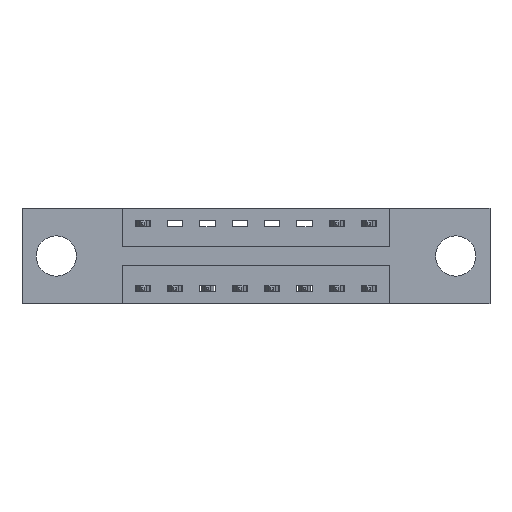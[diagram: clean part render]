
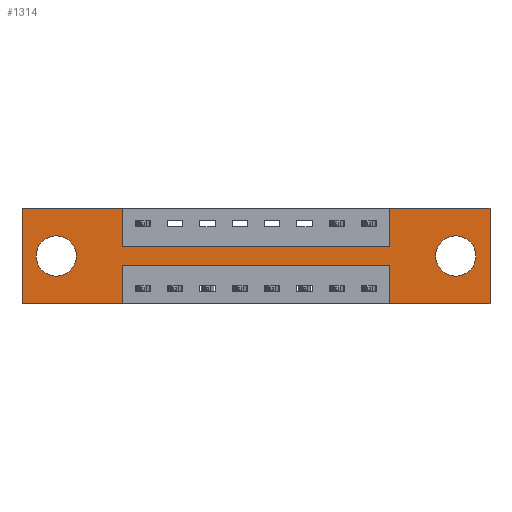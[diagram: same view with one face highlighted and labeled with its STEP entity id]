
A CAD part, front view. The second image highlights one B-rep face of the part: STEP entity #1314.
In plain terms, the highlighted planar face has unit normal (0, -1, 0).
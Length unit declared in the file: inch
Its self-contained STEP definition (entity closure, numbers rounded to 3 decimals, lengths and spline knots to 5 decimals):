
#1 = CARTESIAN_POINT ( 'NONE',  ( 1.4225, 0., 0. ) ) ;
#116 = CARTESIAN_POINT ( 'NONE',  ( 0., 0., 0. ) ) ;
#119 = EDGE_LOOP ( 'NONE', ( #2392, #2402 ) ) ;
#208 = VERTEX_POINT ( 'NONE', #7339 ) ;
#280 = CARTESIAN_POINT ( 'NONE',  ( 1.6775, 0., -0.185 ) ) ;
#337 = DIRECTION ( 'NONE',  ( 0., 1., 0. ) ) ;
#385 = EDGE_LOOP ( 'NONE', ( #2421, #2429, #2489, #2523, #2609, #2802, #2816, #2827, #2843, #3000, #3020, #3051 ) ) ;
#409 = CARTESIAN_POINT ( 'NONE',  ( 1.81, 0., -0.37 ) ) ;
#554 = LINE ( 'NONE', #9428, #5998 ) ;
#558 = DIRECTION ( 'NONE',  ( 0., 0., -1. ) ) ;
#704 = VECTOR ( 'NONE', #7779, 39.37008 ) ;
#785 = VECTOR ( 'NONE', #7935, 39.37008 ) ;
#791 = VERTEX_POINT ( 'NONE', #3571 ) ;
#1025 = CIRCLE ( 'NONE', #1212, 0.078 ) ;
#1055 = VECTOR ( 'NONE', #2573, 39.37008 ) ;
#1145 = CARTESIAN_POINT ( 'NONE',  ( 0.3875, 0., -0.15 ) ) ;
#1210 = DIRECTION ( 'NONE',  ( 0., 0., -1. ) ) ;
#1212 = AXIS2_PLACEMENT_3D ( 'NONE', #280, #5773, #1210 ) ;
#1291 = VECTOR ( 'NONE', #7932, 39.37008 ) ;
#1293 = DIRECTION ( 'NONE',  ( 0., 1., 0. ) ) ;
#1314 = ADVANCED_FACE ( 'NONE', ( #6239, #4576, #6684 ), #6043, .T. ) ;
#1321 = LINE ( 'NONE', #1, #1055 ) ;
#1350 = LINE ( 'NONE', #116, #9336 ) ;
#1404 = VERTEX_POINT ( 'NONE', #4827 ) ;
#1464 = VERTEX_POINT ( 'NONE', #5656 ) ;
#1542 = EDGE_CURVE ( 'NONE', #791, #3186, #3621, .T. ) ;
#1561 = DIRECTION ( 'NONE',  ( 0., -1., 0. ) ) ;
#2259 = ORIENTED_EDGE ( 'NONE', *, *, #2361, .T. ) ;
#2261 = DIRECTION ( 'NONE',  ( 0., 0., -1. ) ) ;
#2269 = VECTOR ( 'NONE', #8347, 39.37008 ) ;
#2274 = VECTOR ( 'NONE', #2781, 39.37008 ) ;
#2292 = AXIS2_PLACEMENT_3D ( 'NONE', #8669, #4455, #9357 ) ;
#2361 = EDGE_CURVE ( 'NONE', #1464, #2610, #3489, .T. ) ;
#2374 = ORIENTED_EDGE ( 'NONE', *, *, #7782, .T. ) ;
#2381 = VECTOR ( 'NONE', #2261, 39.37008 ) ;
#2392 = ORIENTED_EDGE ( 'NONE', *, *, #6526, .T. ) ;
#2402 = ORIENTED_EDGE ( 'NONE', *, *, #7926, .T. ) ;
#2421 = ORIENTED_EDGE ( 'NONE', *, *, #9474, .F. ) ;
#2429 = ORIENTED_EDGE ( 'NONE', *, *, #7641, .F. ) ;
#2475 = VERTEX_POINT ( 'NONE', #8018 ) ;
#2489 = ORIENTED_EDGE ( 'NONE', *, *, #7175, .F. ) ;
#2504 = LINE ( 'NONE', #6474, #2274 ) ;
#2523 = ORIENTED_EDGE ( 'NONE', *, *, #8540, .F. ) ;
#2573 = DIRECTION ( 'NONE',  ( 0., 0., 1. ) ) ;
#2609 = ORIENTED_EDGE ( 'NONE', *, *, #9175, .F. ) ;
#2610 = VERTEX_POINT ( 'NONE', #3074 ) ;
#2759 = CARTESIAN_POINT ( 'NONE',  ( 1.81, 0., 0. ) ) ;
#2781 = DIRECTION ( 'NONE',  ( -1., 0., 0. ) ) ;
#2802 = ORIENTED_EDGE ( 'NONE', *, *, #4690, .F. ) ;
#2816 = ORIENTED_EDGE ( 'NONE', *, *, #6222, .F. ) ;
#2821 = CARTESIAN_POINT ( 'NONE',  ( 0., 0., 0. ) ) ;
#2827 = ORIENTED_EDGE ( 'NONE', *, *, #4799, .F. ) ;
#2843 = ORIENTED_EDGE ( 'NONE', *, *, #3259, .F. ) ;
#2854 = CARTESIAN_POINT ( 'NONE',  ( 0., 0., 0. ) ) ;
#2866 = LINE ( 'NONE', #7402, #2381 ) ;
#2927 = LINE ( 'NONE', #2821, #785 ) ;
#2968 = VERTEX_POINT ( 'NONE', #5697 ) ;
#3000 = ORIENTED_EDGE ( 'NONE', *, *, #5728, .F. ) ;
#3020 = ORIENTED_EDGE ( 'NONE', *, *, #1542, .F. ) ;
#3028 = CIRCLE ( 'NONE', #3893, 0.078 ) ;
#3051 = ORIENTED_EDGE ( 'NONE', *, *, #9039, .F. ) ;
#3074 = CARTESIAN_POINT ( 'NONE',  ( 1.6775, 0., -0.263 ) ) ;
#3094 = CARTESIAN_POINT ( 'NONE',  ( 0., 0., -0.37 ) ) ;
#3111 = VERTEX_POINT ( 'NONE', #7216 ) ;
#3155 = CARTESIAN_POINT ( 'NONE',  ( 1.4225, 0., -0.22 ) ) ;
#3166 = VERTEX_POINT ( 'NONE', #409 ) ;
#3186 = VERTEX_POINT ( 'NONE', #7277 ) ;
#3259 = EDGE_CURVE ( 'NONE', #3849, #1404, #2866, .T. ) ;
#3433 = VERTEX_POINT ( 'NONE', #3155 ) ;
#3489 = CIRCLE ( 'NONE', #5369, 0.078 ) ;
#3571 = CARTESIAN_POINT ( 'NONE',  ( 0., 0., -0.37 ) ) ;
#3621 = LINE ( 'NONE', #2854, #1291 ) ;
#3849 = VERTEX_POINT ( 'NONE', #9514 ) ;
#3867 = VECTOR ( 'NONE', #5836, 39.37008 ) ;
#3893 = AXIS2_PLACEMENT_3D ( 'NONE', #5849, #1293, #6554 ) ;
#4069 = LINE ( 'NONE', #4103, #2269 ) ;
#4100 = VECTOR ( 'NONE', #9129, 39.37008 ) ;
#4103 = CARTESIAN_POINT ( 'NONE',  ( 0., 0., -0.37 ) ) ;
#4308 = CARTESIAN_POINT ( 'NONE',  ( 1.4225, 0., -0.37 ) ) ;
#4327 = EDGE_LOOP ( 'NONE', ( #2259, #2374 ) ) ;
#4455 = DIRECTION ( 'NONE',  ( 0., 1., 0. ) ) ;
#4515 = LINE ( 'NONE', #1145, #8049 ) ;
#4576 = FACE_BOUND ( 'NONE', #119, .T. ) ;
#4690 = EDGE_CURVE ( 'NONE', #2475, #4815, #1350, .T. ) ;
#4799 = EDGE_CURVE ( 'NONE', #1404, #5065, #4515, .T. ) ;
#4815 = VERTEX_POINT ( 'NONE', #2759 ) ;
#4827 = CARTESIAN_POINT ( 'NONE',  ( 0.3875, 0., -0.15 ) ) ;
#5031 = LINE ( 'NONE', #8431, #4100 ) ;
#5065 = VERTEX_POINT ( 'NONE', #7374 ) ;
#5107 = CARTESIAN_POINT ( 'NONE',  ( 1.6775, 0., -0.185 ) ) ;
#5128 = CARTESIAN_POINT ( 'NONE',  ( 1.4225, 0., -0.37 ) ) ;
#5369 = AXIS2_PLACEMENT_3D ( 'NONE', #5107, #337, #5813 ) ;
#5635 = VERTEX_POINT ( 'NONE', #4308 ) ;
#5648 = DIRECTION ( 'NONE',  ( 1., 0., 0. ) ) ;
#5656 = CARTESIAN_POINT ( 'NONE',  ( 1.6775, 0., -0.107 ) ) ;
#5697 = CARTESIAN_POINT ( 'NONE',  ( 0.1325, 0., -0.107 ) ) ;
#5728 = EDGE_CURVE ( 'NONE', #3186, #3849, #2927, .T. ) ;
#5773 = DIRECTION ( 'NONE',  ( 0., 1., 0. ) ) ;
#5813 = DIRECTION ( 'NONE',  ( 0., 0., -1. ) ) ;
#5836 = DIRECTION ( 'NONE',  ( 0., 0., 1. ) ) ;
#5849 = CARTESIAN_POINT ( 'NONE',  ( 0.1325, 0., -0.185 ) ) ;
#5998 = VECTOR ( 'NONE', #558, 39.37008 ) ;
#6035 = LINE ( 'NONE', #5128, #3867 ) ;
#6043 = PLANE ( 'NONE',  #9333 ) ;
#6181 = VERTEX_POINT ( 'NONE', #9668 ) ;
#6222 = EDGE_CURVE ( 'NONE', #5065, #2475, #1321, .T. ) ;
#6239 = FACE_BOUND ( 'NONE', #4327, .T. ) ;
#6474 = CARTESIAN_POINT ( 'NONE',  ( 0., 0., -0.37 ) ) ;
#6526 = EDGE_CURVE ( 'NONE', #2968, #3111, #3028, .T. ) ;
#6554 = DIRECTION ( 'NONE',  ( 0., 0., 1. ) ) ;
#6684 = FACE_OUTER_BOUND ( 'NONE', #385, .T. ) ;
#6777 = LINE ( 'NONE', #7065, #704 ) ;
#6788 = DIRECTION ( 'NONE',  ( 0., 0., -1. ) ) ;
#7065 = CARTESIAN_POINT ( 'NONE',  ( 1.81, 0., 0. ) ) ;
#7175 = EDGE_CURVE ( 'NONE', #5635, #3433, #6035, .T. ) ;
#7216 = CARTESIAN_POINT ( 'NONE',  ( 0.1325, 0., -0.263 ) ) ;
#7277 = CARTESIAN_POINT ( 'NONE',  ( 0., 0., 0. ) ) ;
#7339 = CARTESIAN_POINT ( 'NONE',  ( 0.3875, 0., -0.37 ) ) ;
#7374 = CARTESIAN_POINT ( 'NONE',  ( 1.4225, 0., -0.15 ) ) ;
#7402 = CARTESIAN_POINT ( 'NONE',  ( 0.3875, 0., 0. ) ) ;
#7561 = CIRCLE ( 'NONE', #2292, 0.078 ) ;
#7641 = EDGE_CURVE ( 'NONE', #3433, #6181, #5031, .T. ) ;
#7779 = DIRECTION ( 'NONE',  ( 0., 0., -1. ) ) ;
#7782 = EDGE_CURVE ( 'NONE', #2610, #1464, #1025, .T. ) ;
#7832 = DIRECTION ( 'NONE',  ( 1., 0., 0. ) ) ;
#7926 = EDGE_CURVE ( 'NONE', #3111, #2968, #7561, .T. ) ;
#7932 = DIRECTION ( 'NONE',  ( 0., 0., 1. ) ) ;
#7935 = DIRECTION ( 'NONE',  ( 1., 0., 0. ) ) ;
#8018 = CARTESIAN_POINT ( 'NONE',  ( 1.4225, 0., 0. ) ) ;
#8049 = VECTOR ( 'NONE', #7832, 39.37008 ) ;
#8347 = DIRECTION ( 'NONE',  ( -1., 0., 0. ) ) ;
#8431 = CARTESIAN_POINT ( 'NONE',  ( 0.3875, 0., -0.22 ) ) ;
#8540 = EDGE_CURVE ( 'NONE', #3166, #5635, #2504, .T. ) ;
#8669 = CARTESIAN_POINT ( 'NONE',  ( 0.1325, 0., -0.185 ) ) ;
#9039 = EDGE_CURVE ( 'NONE', #208, #791, #4069, .T. ) ;
#9129 = DIRECTION ( 'NONE',  ( -1., 0., 0. ) ) ;
#9175 = EDGE_CURVE ( 'NONE', #4815, #3166, #6777, .T. ) ;
#9333 = AXIS2_PLACEMENT_3D ( 'NONE', #3094, #1561, #6788 ) ;
#9336 = VECTOR ( 'NONE', #5648, 39.37008 ) ;
#9357 = DIRECTION ( 'NONE',  ( 0., 0., 1. ) ) ;
#9428 = CARTESIAN_POINT ( 'NONE',  ( 0.3875, 0., -0.37 ) ) ;
#9474 = EDGE_CURVE ( 'NONE', #6181, #208, #554, .T. ) ;
#9514 = CARTESIAN_POINT ( 'NONE',  ( 0.3875, 0., 0. ) ) ;
#9668 = CARTESIAN_POINT ( 'NONE',  ( 0.3875, 0., -0.22 ) ) ;
